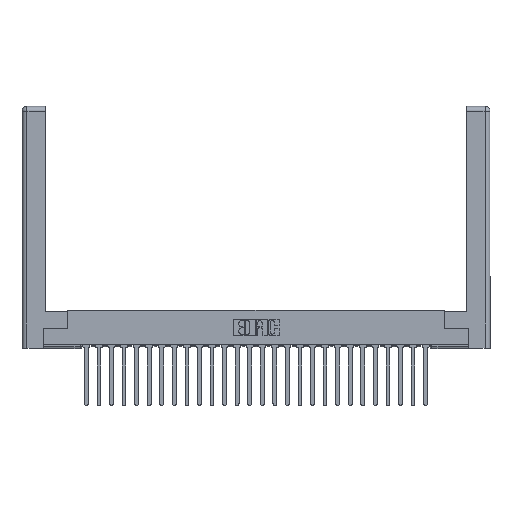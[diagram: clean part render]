
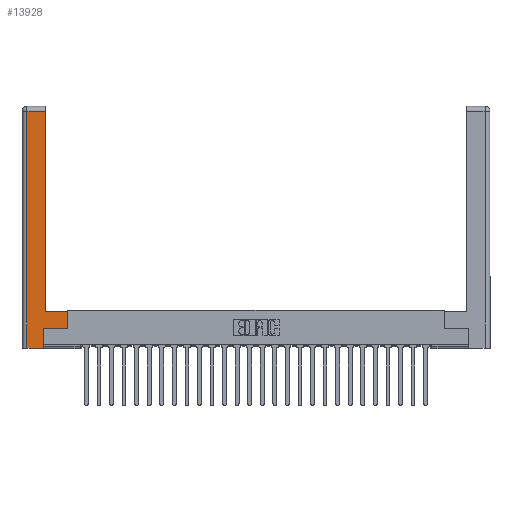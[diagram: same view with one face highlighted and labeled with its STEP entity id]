
A CAD part, top view. The second image highlights one B-rep face of the part: STEP entity #13928.
In plain terms, the highlighted planar face has unit normal (0, 0, 1).
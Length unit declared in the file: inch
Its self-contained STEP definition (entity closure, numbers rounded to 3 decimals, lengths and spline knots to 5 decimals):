
#273 = LINE ( 'NONE', #2652, #9053 ) ;
#562 = VERTEX_POINT ( 'NONE', #8921 ) ;
#683 = LINE ( 'NONE', #9728, #3675 ) ;
#692 = VECTOR ( 'NONE', #2622, 39.37008 ) ;
#1650 = VERTEX_POINT ( 'NONE', #23320 ) ;
#1654 = ORIENTED_EDGE ( 'NONE', *, *, #25985, .T. ) ;
#1809 = EDGE_CURVE ( 'NONE', #10898, #17848, #23757, .T. ) ;
#2599 = DIRECTION ( 'NONE',  ( 0., 0., -1. ) ) ;
#2622 = DIRECTION ( 'NONE',  ( 1., 0., 0. ) ) ;
#2652 = CARTESIAN_POINT ( 'NONE',  ( 0.265, 0.245, 0. ) ) ;
#3377 = ORIENTED_EDGE ( 'NONE', *, *, #16766, .T. ) ;
#3675 = VECTOR ( 'NONE', #18763, 39.37008 ) ;
#3855 = EDGE_CURVE ( 'NONE', #1650, #18346, #27491, .T. ) ;
#4429 = VERTEX_POINT ( 'NONE', #7614 ) ;
#4664 = CARTESIAN_POINT ( 'NONE',  ( 0., 0., 0. ) ) ;
#5265 = VERTEX_POINT ( 'NONE', #9880 ) ;
#5504 = LINE ( 'NONE', #25349, #26146 ) ;
#7614 = CARTESIAN_POINT ( 'NONE',  ( 0.295, 0.45, 0. ) ) ;
#8382 = CARTESIAN_POINT ( 'NONE',  ( 0.295, 3., 0. ) ) ;
#8921 = CARTESIAN_POINT ( 'NONE',  ( 0.565, 0.45, 0. ) ) ;
#8984 = LINE ( 'NONE', #18611, #20660 ) ;
#9053 = VECTOR ( 'NONE', #21016, 39.37008 ) ;
#9728 = CARTESIAN_POINT ( 'NONE',  ( 0.565, 0.245, 0. ) ) ;
#9880 = CARTESIAN_POINT ( 'NONE',  ( 0.565, 0.245, 0. ) ) ;
#10044 = VECTOR ( 'NONE', #16038, 39.37008 ) ;
#10108 = VERTEX_POINT ( 'NONE', #14964 ) ;
#10716 = EDGE_CURVE ( 'NONE', #562, #4429, #13833, .T. ) ;
#10879 = VECTOR ( 'NONE', #19315, 39.37008 ) ;
#10898 = VERTEX_POINT ( 'NONE', #19723 ) ;
#11554 = AXIS2_PLACEMENT_3D ( 'NONE', #4664, #2599, #13738 ) ;
#12604 = ORIENTED_EDGE ( 'NONE', *, *, #19955, .T. ) ;
#12842 = LINE ( 'NONE', #8382, #28202 ) ;
#13043 = EDGE_LOOP ( 'NONE', ( #19656, #25807, #3377, #28672, #22390, #12604, #1654, #17102 ) ) ;
#13738 = DIRECTION ( 'NONE',  ( -1., 0., 0. ) ) ;
#13833 = LINE ( 'NONE', #27279, #10044 ) ;
#13928 = ADVANCED_FACE ( 'NONE', ( #15949 ), #24961, .F. ) ;
#14049 = DIRECTION ( 'NONE',  ( 0., -1., 0. ) ) ;
#14850 = CARTESIAN_POINT ( 'NONE',  ( 0.0615, 2.94, 0. ) ) ;
#14964 = CARTESIAN_POINT ( 'NONE',  ( 0.265, 0.245, 0. ) ) ;
#15949 = FACE_OUTER_BOUND ( 'NONE', #13043, .T. ) ;
#16038 = DIRECTION ( 'NONE',  ( -1., 0., 0. ) ) ;
#16766 = EDGE_CURVE ( 'NONE', #17848, #1650, #8984, .T. ) ;
#17102 = ORIENTED_EDGE ( 'NONE', *, *, #10716, .T. ) ;
#17848 = VERTEX_POINT ( 'NONE', #14850 ) ;
#18045 = CARTESIAN_POINT ( 'NONE',  ( 0.265, 0., 0. ) ) ;
#18346 = VERTEX_POINT ( 'NONE', #22139 ) ;
#18369 = EDGE_CURVE ( 'NONE', #4429, #10898, #12842, .T. ) ;
#18611 = CARTESIAN_POINT ( 'NONE',  ( 0.0615, 0., 0. ) ) ;
#18763 = DIRECTION ( 'NONE',  ( 1., 0., 0. ) ) ;
#19315 = DIRECTION ( 'NONE',  ( -1., 0., 0. ) ) ;
#19464 = CARTESIAN_POINT ( 'NONE',  ( 0.0615, 2.94, 0. ) ) ;
#19656 = ORIENTED_EDGE ( 'NONE', *, *, #18369, .T. ) ;
#19723 = CARTESIAN_POINT ( 'NONE',  ( 0.295, 2.94, 0. ) ) ;
#19955 = EDGE_CURVE ( 'NONE', #10108, #5265, #683, .T. ) ;
#20660 = VECTOR ( 'NONE', #14049, 39.37008 ) ;
#21016 = DIRECTION ( 'NONE',  ( 0., 1., 0. ) ) ;
#21337 = DIRECTION ( 'NONE',  ( 0., 1., 0. ) ) ;
#21849 = DIRECTION ( 'NONE',  ( 0., 1., 0. ) ) ;
#22139 = CARTESIAN_POINT ( 'NONE',  ( 0.265, 0., 0. ) ) ;
#22390 = ORIENTED_EDGE ( 'NONE', *, *, #25104, .T. ) ;
#23320 = CARTESIAN_POINT ( 'NONE',  ( 0.0615, 0., 0. ) ) ;
#23757 = LINE ( 'NONE', #19464, #10879 ) ;
#24961 = PLANE ( 'NONE',  #11554 ) ;
#25104 = EDGE_CURVE ( 'NONE', #18346, #10108, #273, .T. ) ;
#25349 = CARTESIAN_POINT ( 'NONE',  ( 0.565, 0.45, 0. ) ) ;
#25807 = ORIENTED_EDGE ( 'NONE', *, *, #1809, .T. ) ;
#25985 = EDGE_CURVE ( 'NONE', #5265, #562, #5504, .T. ) ;
#26146 = VECTOR ( 'NONE', #21337, 39.37008 ) ;
#27279 = CARTESIAN_POINT ( 'NONE',  ( 0.295, 0.45, 0. ) ) ;
#27491 = LINE ( 'NONE', #18045, #692 ) ;
#28202 = VECTOR ( 'NONE', #21849, 39.37008 ) ;
#28672 = ORIENTED_EDGE ( 'NONE', *, *, #3855, .T. ) ;
